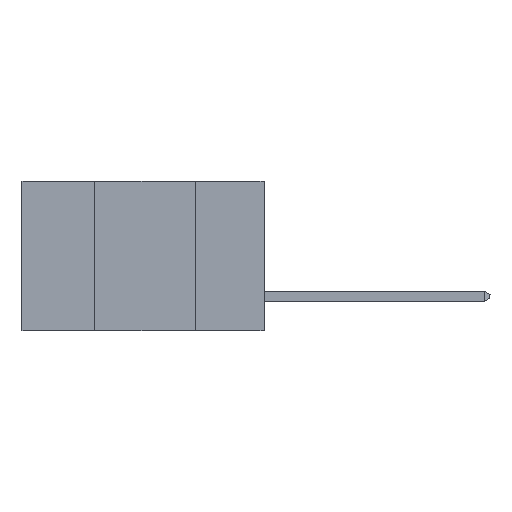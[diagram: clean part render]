
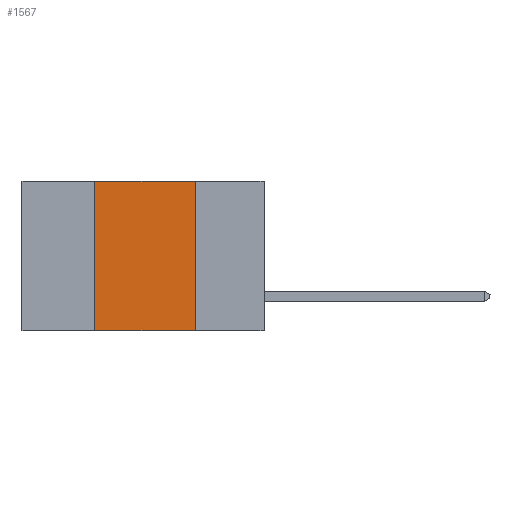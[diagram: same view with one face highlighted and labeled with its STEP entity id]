
A CAD part, left-side view. The second image highlights one B-rep face of the part: STEP entity #1567.
In plain terms, the highlighted planar face has unit normal (-1, 0, 0).
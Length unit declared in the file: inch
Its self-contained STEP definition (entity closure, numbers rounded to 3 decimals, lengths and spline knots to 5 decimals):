
#1567 = ADVANCED_FACE ( 'NONE', ( #8027 ), #23521, .F. ) ;
#2085 = LINE ( 'NONE', #5521, #15791 ) ;
#2157 = EDGE_CURVE ( 'NONE', #8201, #23707, #2085, .T. ) ;
#3181 = CARTESIAN_POINT ( 'NONE',  ( 0., 0.6, 0. ) ) ;
#4347 = AXIS2_PLACEMENT_3D ( 'NONE', #3181, #19883, #9452 ) ;
#4576 = CARTESIAN_POINT ( 'NONE',  ( 0., 0.17, 0. ) ) ;
#5000 = VECTOR ( 'NONE', #5691, 39.37008 ) ;
#5171 = LINE ( 'NONE', #13372, #5000 ) ;
#5521 = CARTESIAN_POINT ( 'NONE',  ( 0., 0.6, 0. ) ) ;
#5641 = CARTESIAN_POINT ( 'NONE',  ( 0., 0.17, -0.37 ) ) ;
#5691 = DIRECTION ( 'NONE',  ( 0., 0., -1. ) ) ;
#6407 = ORIENTED_EDGE ( 'NONE', *, *, #12635, .F. ) ;
#6923 = VERTEX_POINT ( 'NONE', #5641 ) ;
#7184 = ORIENTED_EDGE ( 'NONE', *, *, #10825, .T. ) ;
#7424 = EDGE_CURVE ( 'NONE', #23707, #6923, #5171, .T. ) ;
#8027 = FACE_OUTER_BOUND ( 'NONE', #17412, .T. ) ;
#8201 = VERTEX_POINT ( 'NONE', #12759 ) ;
#9452 = DIRECTION ( 'NONE',  ( 0., 0., -1. ) ) ;
#9691 = VERTEX_POINT ( 'NONE', #19372 ) ;
#10825 = EDGE_CURVE ( 'NONE', #9691, #6923, #22723, .T. ) ;
#10909 = DIRECTION ( 'NONE',  ( 0., -1., 0. ) ) ;
#12635 = EDGE_CURVE ( 'NONE', #9691, #8201, #21510, .T. ) ;
#12759 = CARTESIAN_POINT ( 'NONE',  ( 0., 0.42, 0. ) ) ;
#13372 = CARTESIAN_POINT ( 'NONE',  ( 0., 0.17, 0. ) ) ;
#14947 = DIRECTION ( 'NONE',  ( 0., -1., 0. ) ) ;
#15791 = VECTOR ( 'NONE', #14947, 39.37008 ) ;
#15960 = ORIENTED_EDGE ( 'NONE', *, *, #2157, .F. ) ;
#15970 = ORIENTED_EDGE ( 'NONE', *, *, #7424, .F. ) ;
#16663 = VECTOR ( 'NONE', #20086, 39.37008 ) ;
#17412 = EDGE_LOOP ( 'NONE', ( #15970, #15960, #6407, #7184 ) ) ;
#18198 = CARTESIAN_POINT ( 'NONE',  ( 0., 0.42, 0. ) ) ;
#19372 = CARTESIAN_POINT ( 'NONE',  ( 0., 0.42, -0.37 ) ) ;
#19883 = DIRECTION ( 'NONE',  ( 1., 0., 0. ) ) ;
#19934 = CARTESIAN_POINT ( 'NONE',  ( 0., 0.6, -0.37 ) ) ;
#20086 = DIRECTION ( 'NONE',  ( 0., 0., 1. ) ) ;
#21510 = LINE ( 'NONE', #18198, #16663 ) ;
#22723 = LINE ( 'NONE', #19934, #23589 ) ;
#23521 = PLANE ( 'NONE',  #4347 ) ;
#23589 = VECTOR ( 'NONE', #10909, 39.37008 ) ;
#23707 = VERTEX_POINT ( 'NONE', #4576 ) ;
